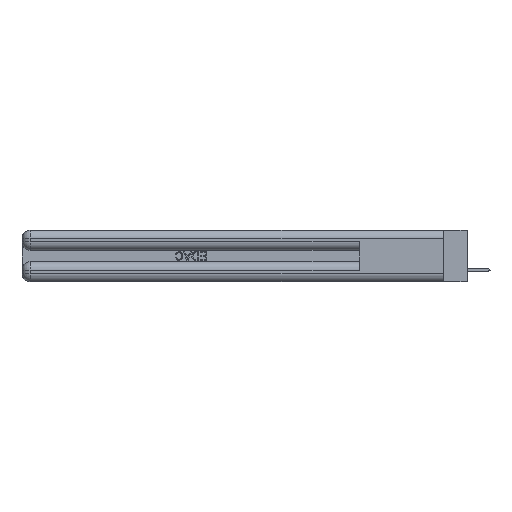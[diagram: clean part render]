
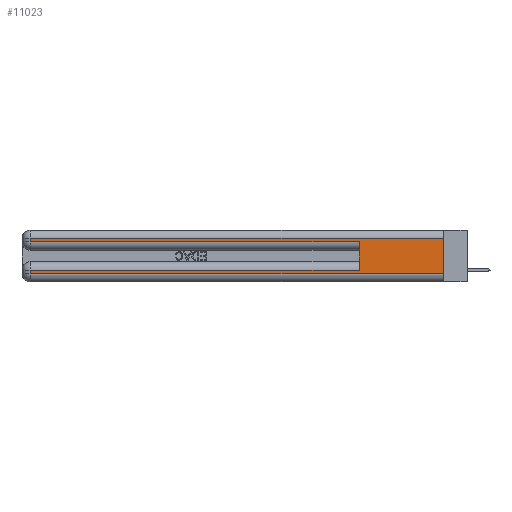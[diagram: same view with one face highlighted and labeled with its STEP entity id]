
A CAD part, left-side view. The second image highlights one B-rep face of the part: STEP entity #11023.
In plain terms, the highlighted planar face has unit normal (-1, 0, 0).
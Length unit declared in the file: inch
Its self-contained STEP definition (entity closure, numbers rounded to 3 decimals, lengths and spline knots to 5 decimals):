
#569 = CARTESIAN_POINT ( 'NONE',  ( 0., 0., 0.06 ) ) ;
#1017 = CARTESIAN_POINT ( 'NONE',  ( 0., 0., 0.31 ) ) ;
#2919 = VERTEX_POINT ( 'NONE', #10888 ) ;
#3154 = LINE ( 'NONE', #15040, #41938 ) ;
#3874 = CARTESIAN_POINT ( 'NONE',  ( 0., 0.6, 0.145 ) ) ;
#4640 = VERTEX_POINT ( 'NONE', #34969 ) ;
#5341 = VECTOR ( 'NONE', #8459, 39.37008 ) ;
#6588 = EDGE_CURVE ( 'NONE', #32752, #4640, #11804, .T. ) ;
#7138 = ORIENTED_EDGE ( 'NONE', *, *, #26416, .T. ) ;
#7308 = EDGE_CURVE ( 'NONE', #27363, #4640, #18595, .T. ) ;
#8459 = DIRECTION ( 'NONE',  ( 0., -1., 0. ) ) ;
#10888 = CARTESIAN_POINT ( 'NONE',  ( 0., 2.94, 0.06 ) ) ;
#10987 = VERTEX_POINT ( 'NONE', #23279 ) ;
#11023 = ADVANCED_FACE ( 'NONE', ( #48294 ), #18254, .F. ) ;
#11083 = VECTOR ( 'NONE', #13061, 39.37008 ) ;
#11655 = DIRECTION ( 'NONE',  ( 0., 0., -1. ) ) ;
#11804 = LINE ( 'NONE', #33948, #39410 ) ;
#12614 = EDGE_CURVE ( 'NONE', #2919, #10987, #18467, .T. ) ;
#12763 = CARTESIAN_POINT ( 'NONE',  ( 0., 2.94, 0.37 ) ) ;
#13061 = DIRECTION ( 'NONE',  ( 0., 1., 0. ) ) ;
#13965 = DIRECTION ( 'NONE',  ( 0., -1., 0. ) ) ;
#14759 = CARTESIAN_POINT ( 'NONE',  ( 0., 0., 0.37 ) ) ;
#15040 = CARTESIAN_POINT ( 'NONE',  ( 0., 2.94, 0.37 ) ) ;
#15705 = LINE ( 'NONE', #14759, #42689 ) ;
#18254 = PLANE ( 'NONE',  #33636 ) ;
#18467 = LINE ( 'NONE', #569, #5341 ) ;
#18595 = LINE ( 'NONE', #3874, #41775 ) ;
#18950 = VERTEX_POINT ( 'NONE', #38521 ) ;
#19954 = ORIENTED_EDGE ( 'NONE', *, *, #6588, .T. ) ;
#21118 = EDGE_CURVE ( 'NONE', #50556, #10987, #15705, .T. ) ;
#21160 = DIRECTION ( 'NONE',  ( 0., 0., -1. ) ) ;
#21166 = ORIENTED_EDGE ( 'NONE', *, *, #7308, .F. ) ;
#22531 = DIRECTION ( 'NONE',  ( 0., 1., 0. ) ) ;
#23279 = CARTESIAN_POINT ( 'NONE',  ( 0., 0., 0.06 ) ) ;
#23396 = DIRECTION ( 'NONE',  ( 0., 0., -1. ) ) ;
#24371 = ORIENTED_EDGE ( 'NONE', *, *, #12614, .T. ) ;
#25894 = CARTESIAN_POINT ( 'NONE',  ( 0., 0.6, 0.085 ) ) ;
#26082 = ORIENTED_EDGE ( 'NONE', *, *, #32904, .T. ) ;
#26416 = EDGE_CURVE ( 'NONE', #50556, #18950, #51127, .T. ) ;
#27363 = VERTEX_POINT ( 'NONE', #25894 ) ;
#27444 = LINE ( 'NONE', #42302, #46136 ) ;
#30411 = VECTOR ( 'NONE', #21160, 39.37008 ) ;
#31037 = ORIENTED_EDGE ( 'NONE', *, *, #43000, .T. ) ;
#31771 = DIRECTION ( 'NONE',  ( 1., 0., 0. ) ) ;
#31862 = DIRECTION ( 'NONE',  ( 0., 0., 1. ) ) ;
#32752 = VERTEX_POINT ( 'NONE', #43663 ) ;
#32904 = EDGE_CURVE ( 'NONE', #27363, #42822, #27444, .T. ) ;
#33636 = AXIS2_PLACEMENT_3D ( 'NONE', #35276, #31771, #11655 ) ;
#33948 = CARTESIAN_POINT ( 'NONE',  ( 0., 0., 0.285 ) ) ;
#34969 = CARTESIAN_POINT ( 'NONE',  ( 0., 0.6, 0.285 ) ) ;
#35276 = CARTESIAN_POINT ( 'NONE',  ( 0., 0., 0.37 ) ) ;
#35964 = ORIENTED_EDGE ( 'NONE', *, *, #45717, .T. ) ;
#38521 = CARTESIAN_POINT ( 'NONE',  ( 0., 2.94, 0.31 ) ) ;
#39410 = VECTOR ( 'NONE', #13965, 39.37008 ) ;
#39437 = DIRECTION ( 'NONE',  ( 0., 0., -1. ) ) ;
#41775 = VECTOR ( 'NONE', #31862, 39.37008 ) ;
#41938 = VECTOR ( 'NONE', #39437, 39.37008 ) ;
#42302 = CARTESIAN_POINT ( 'NONE',  ( 0., 0., 0.085 ) ) ;
#42689 = VECTOR ( 'NONE', #23396, 39.37008 ) ;
#42822 = VERTEX_POINT ( 'NONE', #46964 ) ;
#43000 = EDGE_CURVE ( 'NONE', #18950, #32752, #43545, .T. ) ;
#43545 = LINE ( 'NONE', #12763, #30411 ) ;
#43663 = CARTESIAN_POINT ( 'NONE',  ( 0., 2.94, 0.285 ) ) ;
#45717 = EDGE_CURVE ( 'NONE', #42822, #2919, #3154, .T. ) ;
#46136 = VECTOR ( 'NONE', #22531, 39.37008 ) ;
#46625 = EDGE_LOOP ( 'NONE', ( #51418, #7138, #31037, #19954, #21166, #26082, #35964, #24371 ) ) ;
#46964 = CARTESIAN_POINT ( 'NONE',  ( 0., 2.94, 0.085 ) ) ;
#48294 = FACE_OUTER_BOUND ( 'NONE', #46625, .T. ) ;
#50556 = VERTEX_POINT ( 'NONE', #51810 ) ;
#51127 = LINE ( 'NONE', #1017, #11083 ) ;
#51418 = ORIENTED_EDGE ( 'NONE', *, *, #21118, .F. ) ;
#51810 = CARTESIAN_POINT ( 'NONE',  ( 0., 0., 0.31 ) ) ;
